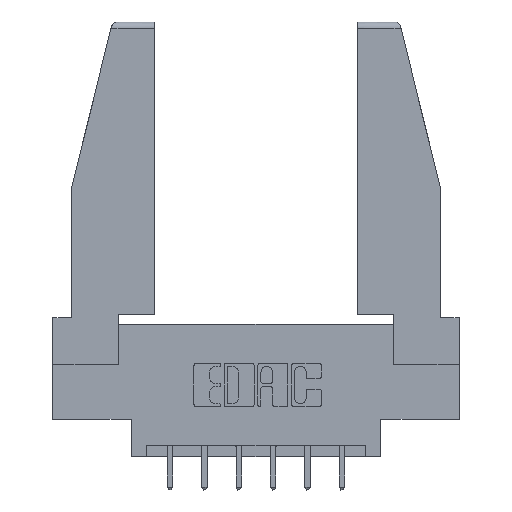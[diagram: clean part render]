
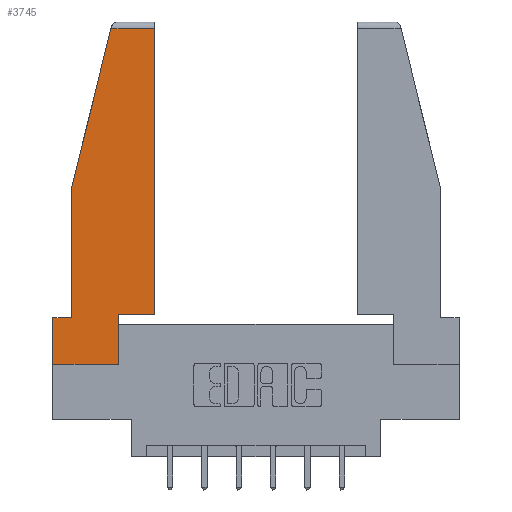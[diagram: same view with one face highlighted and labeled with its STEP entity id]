
A CAD part, top view. The second image highlights one B-rep face of the part: STEP entity #3745.
In plain terms, the highlighted planar face has unit normal (0, 0, 1).
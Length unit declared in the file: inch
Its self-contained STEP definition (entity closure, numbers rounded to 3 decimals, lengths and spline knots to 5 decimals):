
#5 = DIRECTION ( 'NONE',  ( 0., -1., 0. ) ) ;
#7 = DIRECTION ( 'NONE',  ( 0., 1., 0. ) ) ;
#29 = DIRECTION ( 'NONE',  ( 0., 1., 0. ) ) ;
#164 = LINE ( 'NONE', #3837, #4914 ) ;
#320 = VECTOR ( 'NONE', #9124, 39.37008 ) ;
#372 = VECTOR ( 'NONE', #2172, 39.37008 ) ;
#510 = EDGE_LOOP ( 'NONE', ( #1689, #1181, #10588, #6570, #1647, #7423, #1366, #4410, #10844 ) ) ;
#875 = DIRECTION ( 'NONE',  ( 0., -1., 0. ) ) ;
#1022 = CARTESIAN_POINT ( 'NONE',  ( 0.461, 0.223, 0. ) ) ;
#1149 = VECTOR ( 'NONE', #875, 39.37008 ) ;
#1181 = ORIENTED_EDGE ( 'NONE', *, *, #7346, .T. ) ;
#1282 = VECTOR ( 'NONE', #7, 39.37008 ) ;
#1314 = VERTEX_POINT ( 'NONE', #10395 ) ;
#1366 = ORIENTED_EDGE ( 'NONE', *, *, #4150, .T. ) ;
#1647 = ORIENTED_EDGE ( 'NONE', *, *, #7298, .T. ) ;
#1677 = CARTESIAN_POINT ( 'NONE',  ( 0.086, 0.8, 0. ) ) ;
#1689 = ORIENTED_EDGE ( 'NONE', *, *, #6008, .T. ) ;
#1867 = CARTESIAN_POINT ( 'NONE',  ( 0.086, 0.21, 0. ) ) ;
#2172 = DIRECTION ( 'NONE',  ( -1., 0., 0. ) ) ;
#2230 = CARTESIAN_POINT ( 'NONE',  ( 0.461, 1.52, 0. ) ) ;
#2294 = EDGE_CURVE ( 'NONE', #8805, #1314, #3724, .T. ) ;
#2458 = VERTEX_POINT ( 'NONE', #4585 ) ;
#2680 = CARTESIAN_POINT ( 'NONE',  ( 0., 0.21, 0. ) ) ;
#2776 = AXIS2_PLACEMENT_3D ( 'NONE', #4819, #4700, #4776 ) ;
#3038 = DIRECTION ( 'NONE',  ( -0.239, -0.971, 0. ) ) ;
#3125 = CARTESIAN_POINT ( 'NONE',  ( 0., 0., 0. ) ) ;
#3354 = VERTEX_POINT ( 'NONE', #5490 ) ;
#3724 = LINE ( 'NONE', #5849, #5737 ) ;
#3745 = ADVANCED_FACE ( 'NONE', ( #11743 ), #9373, .T. ) ;
#3837 = CARTESIAN_POINT ( 'NONE',  ( 0.271, 1.55, 0. ) ) ;
#3874 = VERTEX_POINT ( 'NONE', #3125 ) ;
#4150 = EDGE_CURVE ( 'NONE', #3874, #8805, #9054, .T. ) ;
#4177 = CARTESIAN_POINT ( 'NONE',  ( 0., 0.21, 0. ) ) ;
#4259 = VECTOR ( 'NONE', #5896, 39.37008 ) ;
#4410 = ORIENTED_EDGE ( 'NONE', *, *, #2294, .T. ) ;
#4493 = EDGE_CURVE ( 'NONE', #4728, #3874, #9914, .T. ) ;
#4585 = CARTESIAN_POINT ( 'NONE',  ( 0.2636, 1.52, 0. ) ) ;
#4700 = DIRECTION ( 'NONE',  ( 0., 0., 1. ) ) ;
#4728 = VERTEX_POINT ( 'NONE', #10760 ) ;
#4776 = DIRECTION ( 'NONE',  ( 1., 0., 0. ) ) ;
#4819 = CARTESIAN_POINT ( 'NONE',  ( 0., 0., 0. ) ) ;
#4914 = VECTOR ( 'NONE', #3038, 39.37008 ) ;
#5078 = CARTESIAN_POINT ( 'NONE',  ( 0., 0., 0. ) ) ;
#5267 = VERTEX_POINT ( 'NONE', #2230 ) ;
#5490 = CARTESIAN_POINT ( 'NONE',  ( 0.461, 0.223, 0. ) ) ;
#5693 = LINE ( 'NONE', #4177, #372 ) ;
#5737 = VECTOR ( 'NONE', #29, 39.37008 ) ;
#5824 = VECTOR ( 'NONE', #5, 39.37008 ) ;
#5849 = CARTESIAN_POINT ( 'NONE',  ( 0.297, 0., 0. ) ) ;
#5896 = DIRECTION ( 'NONE',  ( -1., 0., 0. ) ) ;
#6008 = EDGE_CURVE ( 'NONE', #3354, #5267, #7754, .T. ) ;
#6346 = VERTEX_POINT ( 'NONE', #1867 ) ;
#6570 = ORIENTED_EDGE ( 'NONE', *, *, #8082, .T. ) ;
#6649 = CARTESIAN_POINT ( 'NONE',  ( 0.297, 0., 0. ) ) ;
#7298 = EDGE_CURVE ( 'NONE', #6346, #4728, #5693, .T. ) ;
#7346 = EDGE_CURVE ( 'NONE', #5267, #2458, #8875, .T. ) ;
#7423 = ORIENTED_EDGE ( 'NONE', *, *, #4493, .T. ) ;
#7441 = CARTESIAN_POINT ( 'NONE',  ( 0.297, 0.223, 0. ) ) ;
#7754 = LINE ( 'NONE', #1022, #1282 ) ;
#8082 = EDGE_CURVE ( 'NONE', #10498, #6346, #11717, .T. ) ;
#8344 = CARTESIAN_POINT ( 'NONE',  ( 0.086, 0.8, 0. ) ) ;
#8805 = VERTEX_POINT ( 'NONE', #6649 ) ;
#8875 = LINE ( 'NONE', #11532, #4259 ) ;
#9054 = LINE ( 'NONE', #5078, #11220 ) ;
#9124 = DIRECTION ( 'NONE',  ( 1., 0., 0. ) ) ;
#9371 = EDGE_CURVE ( 'NONE', #1314, #3354, #9954, .T. ) ;
#9373 = PLANE ( 'NONE',  #2776 ) ;
#9487 = EDGE_CURVE ( 'NONE', #2458, #10498, #164, .T. ) ;
#9914 = LINE ( 'NONE', #2680, #1149 ) ;
#9954 = LINE ( 'NONE', #7441, #320 ) ;
#10395 = CARTESIAN_POINT ( 'NONE',  ( 0.297, 0.223, 0. ) ) ;
#10494 = DIRECTION ( 'NONE',  ( 1., 0., 0. ) ) ;
#10498 = VERTEX_POINT ( 'NONE', #1677 ) ;
#10588 = ORIENTED_EDGE ( 'NONE', *, *, #9487, .T. ) ;
#10760 = CARTESIAN_POINT ( 'NONE',  ( 0., 0.21, 0. ) ) ;
#10844 = ORIENTED_EDGE ( 'NONE', *, *, #9371, .T. ) ;
#11220 = VECTOR ( 'NONE', #10494, 39.37008 ) ;
#11532 = CARTESIAN_POINT ( 'NONE',  ( 0., 1.52, 0. ) ) ;
#11717 = LINE ( 'NONE', #8344, #5824 ) ;
#11743 = FACE_OUTER_BOUND ( 'NONE', #510, .T. ) ;
